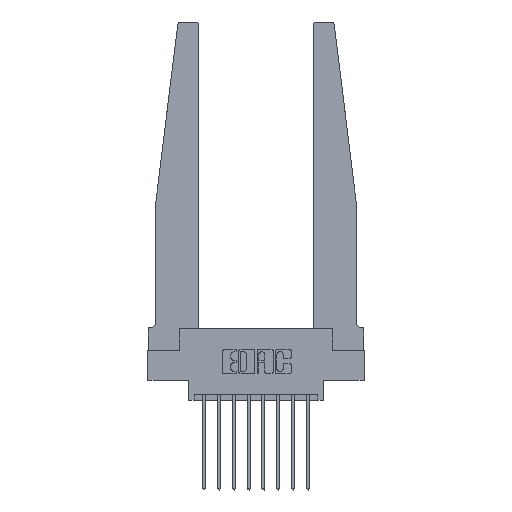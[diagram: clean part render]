
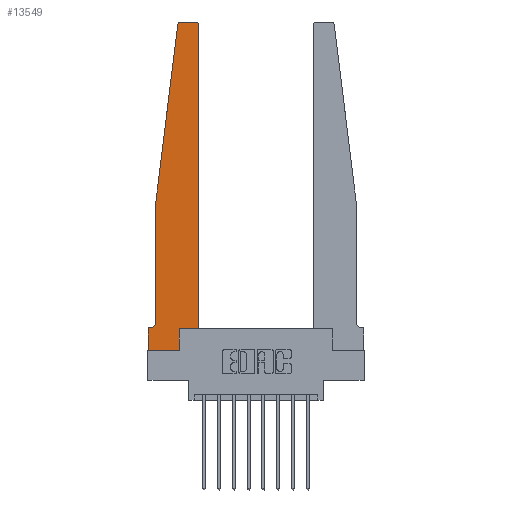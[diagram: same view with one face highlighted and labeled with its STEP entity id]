
A CAD part, top view. The second image highlights one B-rep face of the part: STEP entity #13549.
In plain terms, the highlighted planar face has unit normal (0, 0, 1).
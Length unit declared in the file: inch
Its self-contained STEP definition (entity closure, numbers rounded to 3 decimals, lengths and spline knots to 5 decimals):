
#59 = DIRECTION ( 'NONE',  ( 0., 1., 0. ) ) ;
#80 = CARTESIAN_POINT ( 'NONE',  ( 0.065, 0.1875, 0.37 ) ) ;
#756 = CARTESIAN_POINT ( 'NONE',  ( 0.25, 2.75, 0.37 ) ) ;
#846 = LINE ( 'NONE', #13324, #12556 ) ;
#885 = VECTOR ( 'NONE', #3967, 39.37008 ) ;
#894 = ORIENTED_EDGE ( 'NONE', *, *, #10629, .T. ) ;
#1089 = CARTESIAN_POINT ( 'NONE',  ( 0., 0., 0.37 ) ) ;
#1689 = AXIS2_PLACEMENT_3D ( 'NONE', #2387, #10343, #3526 ) ;
#1748 = ORIENTED_EDGE ( 'NONE', *, *, #10539, .T. ) ;
#2146 = VERTEX_POINT ( 'NONE', #12883 ) ;
#2311 = ORIENTED_EDGE ( 'NONE', *, *, #14277, .T. ) ;
#2387 = CARTESIAN_POINT ( 'NONE',  ( 0.015, 0.2375, 0.37 ) ) ;
#2696 = VERTEX_POINT ( 'NONE', #10947 ) ;
#2837 = LINE ( 'NONE', #6688, #5830 ) ;
#2990 = ORIENTED_EDGE ( 'NONE', *, *, #6103, .T. ) ;
#3024 = DIRECTION ( 'NONE',  ( 0., 0., 1. ) ) ;
#3091 = DIRECTION ( 'NONE',  ( 0., 0., 1. ) ) ;
#3367 = VERTEX_POINT ( 'NONE', #9899 ) ;
#3526 = DIRECTION ( 'NONE',  ( -1., 0., 0. ) ) ;
#3892 = LINE ( 'NONE', #6389, #9610 ) ;
#3901 = VERTEX_POINT ( 'NONE', #8682 ) ;
#3937 = EDGE_CURVE ( 'NONE', #12839, #3901, #8994, .T. ) ;
#3967 = DIRECTION ( 'NONE',  ( -0.122, -0.992, 0. ) ) ;
#4267 = ORIENTED_EDGE ( 'NONE', *, *, #11238, .T. ) ;
#4382 = VECTOR ( 'NONE', #13711, 39.37008 ) ;
#4408 = CARTESIAN_POINT ( 'NONE',  ( 0., 0.1875, 0.37 ) ) ;
#4448 = CARTESIAN_POINT ( 'NONE',  ( 0.065, 0.2375, 0.37 ) ) ;
#4601 = EDGE_CURVE ( 'NONE', #3901, #14033, #7383, .T. ) ;
#4737 = VERTEX_POINT ( 'NONE', #13451 ) ;
#5006 = VERTEX_POINT ( 'NONE', #12739 ) ;
#5526 = CIRCLE ( 'NONE', #11106, 0.03 ) ;
#5550 = DIRECTION ( 'NONE',  ( 1., 0., 0. ) ) ;
#5636 = ORIENTED_EDGE ( 'NONE', *, *, #13950, .T. ) ;
#5830 = VECTOR ( 'NONE', #14632, 39.37008 ) ;
#5855 = FACE_OUTER_BOUND ( 'NONE', #6091, .T. ) ;
#5876 = EDGE_CURVE ( 'NONE', #8441, #11230, #846, .T. ) ;
#6042 = LINE ( 'NONE', #1089, #12096 ) ;
#6091 = EDGE_LOOP ( 'NONE', ( #11350, #6225, #5636, #6568, #894, #2990, #4267, #12397, #10680, #6704, #2311, #1748 ) ) ;
#6103 = EDGE_CURVE ( 'NONE', #10350, #11902, #7054, .T. ) ;
#6225 = ORIENTED_EDGE ( 'NONE', *, *, #4601, .T. ) ;
#6313 = VECTOR ( 'NONE', #8732, 39.37008 ) ;
#6389 = CARTESIAN_POINT ( 'NONE',  ( 0., 0., 0.37 ) ) ;
#6568 = ORIENTED_EDGE ( 'NONE', *, *, #5876, .T. ) ;
#6688 = CARTESIAN_POINT ( 'NONE',  ( 0.2605, 0.18, 0.37 ) ) ;
#6704 = ORIENTED_EDGE ( 'NONE', *, *, #10763, .T. ) ;
#6950 = AXIS2_PLACEMENT_3D ( 'NONE', #4408, #12356, #5550 ) ;
#7054 = LINE ( 'NONE', #80, #4382 ) ;
#7383 = CIRCLE ( 'NONE', #8930, 0.03 ) ;
#8045 = CARTESIAN_POINT ( 'NONE',  ( 0.425, 0.18, 0.37 ) ) ;
#8441 = VERTEX_POINT ( 'NONE', #11600 ) ;
#8502 = CARTESIAN_POINT ( 'NONE',  ( 0.065, 1.25, 0.37 ) ) ;
#8682 = CARTESIAN_POINT ( 'NONE',  ( 0.27653, 2.75, 0.37 ) ) ;
#8732 = DIRECTION ( 'NONE',  ( -1., 0., 0. ) ) ;
#8766 = VECTOR ( 'NONE', #9413, 39.37008 ) ;
#8800 = CARTESIAN_POINT ( 'NONE',  ( 0.24675, 2.72367, 0.37 ) ) ;
#8860 = CARTESIAN_POINT ( 'NONE',  ( 0., 0.1875, 0.37 ) ) ;
#8930 = AXIS2_PLACEMENT_3D ( 'NONE', #9842, #3024, #10971 ) ;
#8957 = PLANE ( 'NONE',  #6950 ) ;
#8994 = LINE ( 'NONE', #756, #6313 ) ;
#9413 = DIRECTION ( 'NONE',  ( 1., 0., 0. ) ) ;
#9526 = CARTESIAN_POINT ( 'NONE',  ( 0.015, 0.1875, 0.37 ) ) ;
#9610 = VECTOR ( 'NONE', #13204, 39.37008 ) ;
#9842 = CARTESIAN_POINT ( 'NONE',  ( 0.27653, 2.72, 0.37 ) ) ;
#9899 = CARTESIAN_POINT ( 'NONE',  ( 0.425, 0.18, 0.37 ) ) ;
#9909 = CARTESIAN_POINT ( 'NONE',  ( 0.395, 2.72, 0.37 ) ) ;
#9965 = LINE ( 'NONE', #8502, #885 ) ;
#10166 = CIRCLE ( 'NONE', #1689, 0.05 ) ;
#10183 = DIRECTION ( 'NONE',  ( 0., -1., 0. ) ) ;
#10343 = DIRECTION ( 'NONE',  ( 0., 0., -1. ) ) ;
#10350 = VERTEX_POINT ( 'NONE', #9526 ) ;
#10539 = EDGE_CURVE ( 'NONE', #2146, #12839, #5526, .T. ) ;
#10629 = EDGE_CURVE ( 'NONE', #11230, #10350, #10166, .T. ) ;
#10680 = ORIENTED_EDGE ( 'NONE', *, *, #11955, .T. ) ;
#10763 = EDGE_CURVE ( 'NONE', #4737, #3367, #14414, .T. ) ;
#10947 = CARTESIAN_POINT ( 'NONE',  ( 0.2605, 0., 0.37 ) ) ;
#10971 = DIRECTION ( 'NONE',  ( 1., 0., 0. ) ) ;
#11041 = DIRECTION ( 'NONE',  ( 1., 0., 0. ) ) ;
#11106 = AXIS2_PLACEMENT_3D ( 'NONE', #9909, #3091, #11041 ) ;
#11230 = VERTEX_POINT ( 'NONE', #4448 ) ;
#11238 = EDGE_CURVE ( 'NONE', #11902, #5006, #6042, .T. ) ;
#11350 = ORIENTED_EDGE ( 'NONE', *, *, #3937, .T. ) ;
#11357 = VECTOR ( 'NONE', #59, 39.37008 ) ;
#11600 = CARTESIAN_POINT ( 'NONE',  ( 0.065, 1.25, 0.37 ) ) ;
#11902 = VERTEX_POINT ( 'NONE', #8860 ) ;
#11955 = EDGE_CURVE ( 'NONE', #2696, #4737, #2837, .T. ) ;
#12077 = LINE ( 'NONE', #8045, #11357 ) ;
#12096 = VECTOR ( 'NONE', #10183, 39.37008 ) ;
#12356 = DIRECTION ( 'NONE',  ( 0., 0., 1. ) ) ;
#12397 = ORIENTED_EDGE ( 'NONE', *, *, #14425, .T. ) ;
#12556 = VECTOR ( 'NONE', #14456, 39.37008 ) ;
#12739 = CARTESIAN_POINT ( 'NONE',  ( 0., 0., 0.37 ) ) ;
#12814 = CARTESIAN_POINT ( 'NONE',  ( 0.425, 0.18, 0.37 ) ) ;
#12839 = VERTEX_POINT ( 'NONE', #13333 ) ;
#12883 = CARTESIAN_POINT ( 'NONE',  ( 0.425, 2.72, 0.37 ) ) ;
#13204 = DIRECTION ( 'NONE',  ( 1., 0., 0. ) ) ;
#13324 = CARTESIAN_POINT ( 'NONE',  ( 0.065, 1.25, 0.37 ) ) ;
#13333 = CARTESIAN_POINT ( 'NONE',  ( 0.395, 2.75, 0.37 ) ) ;
#13451 = CARTESIAN_POINT ( 'NONE',  ( 0.2605, 0.18, 0.37 ) ) ;
#13549 = ADVANCED_FACE ( 'NONE', ( #5855 ), #8957, .T. ) ;
#13711 = DIRECTION ( 'NONE',  ( -1., 0., 0. ) ) ;
#13950 = EDGE_CURVE ( 'NONE', #14033, #8441, #9965, .T. ) ;
#14033 = VERTEX_POINT ( 'NONE', #8800 ) ;
#14277 = EDGE_CURVE ( 'NONE', #3367, #2146, #12077, .T. ) ;
#14414 = LINE ( 'NONE', #12814, #8766 ) ;
#14425 = EDGE_CURVE ( 'NONE', #5006, #2696, #3892, .T. ) ;
#14456 = DIRECTION ( 'NONE',  ( 0., -1., 0. ) ) ;
#14632 = DIRECTION ( 'NONE',  ( 0., 1., 0. ) ) ;
